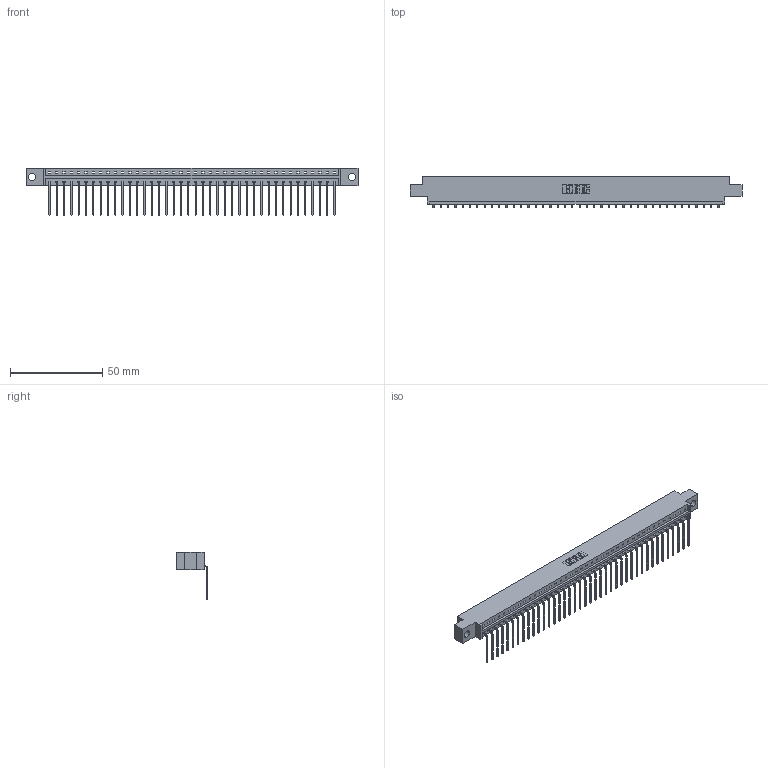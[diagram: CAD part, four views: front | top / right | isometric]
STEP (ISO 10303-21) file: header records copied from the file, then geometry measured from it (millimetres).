
FILE_DESCRIPTION (( 'STEP AP203' ), '1' );
FILE_NAME ('833-040-559-604.STEP', '2020-06-03T18:15:24', ( '' ), ( '' ), 'SwSTEP 2.0', 'SolidWorks 2020', '' );
FILE_SCHEMA (( 'CONFIG_CONTROL_DESIGN' ));
Length unit declared in the file: inch
Products named in the file (3): 345-292-001_558 559 Tail - 1; 833-040-559-604; 833 Part_Offset - .156 Dia - TH
Assembly tree (41 placements, depth 2):
  833-040-559-604
    833 Part_Offset - .156 Dia - TH
    345-292-001_558 559 Tail - 1  x40
Bounding box: 180.04 x 17.09 x 25.53 mm (x, y, z)
Volume: 17917 mm3; surface area: 20183.5 mm2
Topology: 41 solids, 41 shells, 2518 faces, 7603 edges, 5014 vertices
Faces by surface type: plane 1834, cylinder 684
Entity records: 24931 total; most frequent: CARTESIAN_POINT 4310, ORIENTED_EDGE 4286, DIRECTION 3639, EDGE_CURVE 2143, LINE 2015, VECTOR 2015, VERTEX_POINT 1426, AXIS2_PLACEMENT_3D 812
